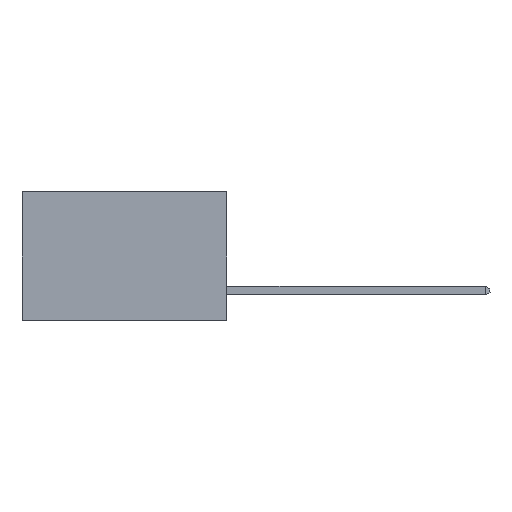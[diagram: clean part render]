
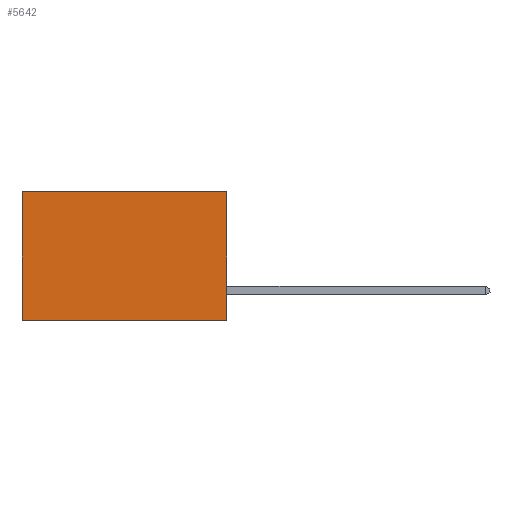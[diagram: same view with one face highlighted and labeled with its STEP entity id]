
A CAD part, left-side view. The second image highlights one B-rep face of the part: STEP entity #5642.
In plain terms, the highlighted planar face has unit normal (-1, 0, 0).
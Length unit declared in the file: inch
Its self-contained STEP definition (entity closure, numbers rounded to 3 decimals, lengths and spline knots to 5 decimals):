
#77 = VERTEX_POINT ( 'NONE', #4505 ) ;
#240 = LINE ( 'NONE', #7672, #5525 ) ;
#273 = CARTESIAN_POINT ( 'NONE',  ( 0.277, 0., -0.37 ) ) ;
#286 = DIRECTION ( 'NONE',  ( 0., 1., 0. ) ) ;
#314 = EDGE_CURVE ( 'NONE', #77, #1439, #240, .T. ) ;
#935 = VECTOR ( 'NONE', #2429, 39.37008 ) ;
#1063 = DIRECTION ( 'NONE',  ( 0., 0., -1. ) ) ;
#1091 = DIRECTION ( 'NONE',  ( 1., 0., 0. ) ) ;
#1118 = PLANE ( 'NONE',  #2025 ) ;
#1170 = EDGE_LOOP ( 'NONE', ( #8408, #1640, #3401, #5150 ) ) ;
#1439 = VERTEX_POINT ( 'NONE', #2209 ) ;
#1640 = ORIENTED_EDGE ( 'NONE', *, *, #5122, .F. ) ;
#1774 = EDGE_CURVE ( 'NONE', #77, #4527, #6262, .T. ) ;
#1776 = CARTESIAN_POINT ( 'NONE',  ( 0.277, 0., -0.37 ) ) ;
#2025 = AXIS2_PLACEMENT_3D ( 'NONE', #1776, #1091, #1063 ) ;
#2209 = CARTESIAN_POINT ( 'NONE',  ( 0.277, 0.59, 0. ) ) ;
#2244 = VERTEX_POINT ( 'NONE', #7857 ) ;
#2429 = DIRECTION ( 'NONE',  ( 0., 0., -1. ) ) ;
#2463 = CARTESIAN_POINT ( 'NONE',  ( 0.277, 0.59, -0.37 ) ) ;
#2512 = VECTOR ( 'NONE', #286, 39.37008 ) ;
#2721 = VECTOR ( 'NONE', #4351, 39.37008 ) ;
#2868 = CARTESIAN_POINT ( 'NONE',  ( 0.277, 0., -0.37 ) ) ;
#3401 = ORIENTED_EDGE ( 'NONE', *, *, #1774, .F. ) ;
#4351 = DIRECTION ( 'NONE',  ( 0., 0., -1. ) ) ;
#4505 = CARTESIAN_POINT ( 'NONE',  ( 0.277, 0., 0. ) ) ;
#4527 = VERTEX_POINT ( 'NONE', #2868 ) ;
#5122 = EDGE_CURVE ( 'NONE', #4527, #2244, #6037, .T. ) ;
#5150 = ORIENTED_EDGE ( 'NONE', *, *, #314, .T. ) ;
#5525 = VECTOR ( 'NONE', #5763, 39.37008 ) ;
#5642 = ADVANCED_FACE ( 'NONE', ( #6967 ), #1118, .F. ) ;
#5763 = DIRECTION ( 'NONE',  ( 0., 1., 0. ) ) ;
#5967 = CARTESIAN_POINT ( 'NONE',  ( 0.277, 0., -0.37 ) ) ;
#6037 = LINE ( 'NONE', #273, #2512 ) ;
#6191 = EDGE_CURVE ( 'NONE', #1439, #2244, #6237, .T. ) ;
#6237 = LINE ( 'NONE', #2463, #935 ) ;
#6262 = LINE ( 'NONE', #5967, #2721 ) ;
#6967 = FACE_OUTER_BOUND ( 'NONE', #1170, .T. ) ;
#7672 = CARTESIAN_POINT ( 'NONE',  ( 0.277, 0., 0. ) ) ;
#7857 = CARTESIAN_POINT ( 'NONE',  ( 0.277, 0.59, -0.37 ) ) ;
#8408 = ORIENTED_EDGE ( 'NONE', *, *, #6191, .T. ) ;
